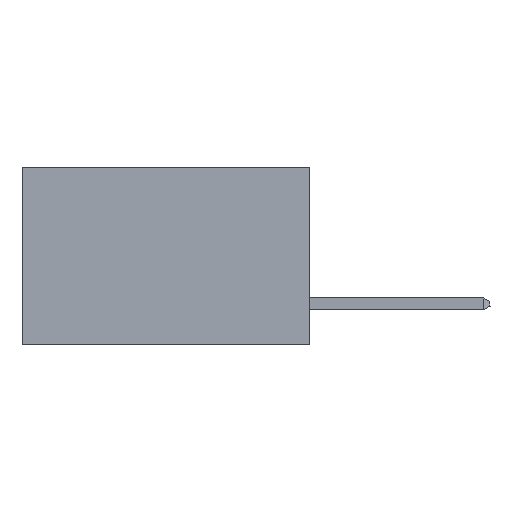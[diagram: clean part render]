
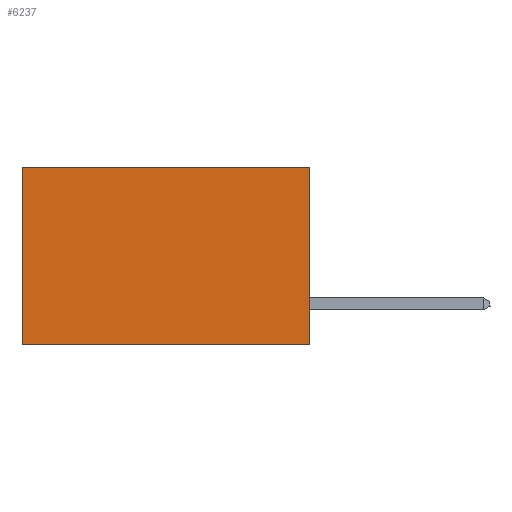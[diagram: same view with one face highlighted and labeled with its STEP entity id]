
A CAD part, left-side view. The second image highlights one B-rep face of the part: STEP entity #6237.
In plain terms, the highlighted planar face has unit normal (-1, 0, 0).
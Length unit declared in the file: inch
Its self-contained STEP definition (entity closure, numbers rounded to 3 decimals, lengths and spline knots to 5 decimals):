
#735 = EDGE_LOOP ( 'NONE', ( #9294, #25639, #48773, #8021 ) ) ;
#2298 = CARTESIAN_POINT ( 'NONE',  ( 0.2875, 0.6, -0.37 ) ) ;
#2796 = CARTESIAN_POINT ( 'NONE',  ( 0.2875, 0., 0. ) ) ;
#3446 = DIRECTION ( 'NONE',  ( 0., 0., -1. ) ) ;
#3773 = PLANE ( 'NONE',  #8908 ) ;
#4714 = LINE ( 'NONE', #18175, #43325 ) ;
#6237 = ADVANCED_FACE ( 'NONE', ( #45340 ), #3773, .F. ) ;
#6367 = CARTESIAN_POINT ( 'NONE',  ( 0.2875, 0.6, 0. ) ) ;
#7957 = CARTESIAN_POINT ( 'NONE',  ( 0.2875, 0., 0. ) ) ;
#8021 = ORIENTED_EDGE ( 'NONE', *, *, #8168, .T. ) ;
#8168 = EDGE_CURVE ( 'NONE', #41315, #24216, #46345, .T. ) ;
#8908 = AXIS2_PLACEMENT_3D ( 'NONE', #7957, #26553, #3446 ) ;
#9294 = ORIENTED_EDGE ( 'NONE', *, *, #49239, .T. ) ;
#15207 = EDGE_CURVE ( 'NONE', #41315, #23271, #4714, .T. ) ;
#16881 = CARTESIAN_POINT ( 'NONE',  ( 0.2875, 0., -0.37 ) ) ;
#17269 = EDGE_CURVE ( 'NONE', #23271, #26229, #37807, .T. ) ;
#18175 = CARTESIAN_POINT ( 'NONE',  ( 0.2875, 0., 0. ) ) ;
#21041 = VECTOR ( 'NONE', #29805, 39.37008 ) ;
#23271 = VERTEX_POINT ( 'NONE', #16881 ) ;
#24216 = VERTEX_POINT ( 'NONE', #43017 ) ;
#25639 = ORIENTED_EDGE ( 'NONE', *, *, #17269, .F. ) ;
#26229 = VERTEX_POINT ( 'NONE', #2298 ) ;
#26553 = DIRECTION ( 'NONE',  ( 1., 0., 0. ) ) ;
#29395 = LINE ( 'NONE', #6367, #34825 ) ;
#29805 = DIRECTION ( 'NONE',  ( 0., 1., 0. ) ) ;
#30519 = CARTESIAN_POINT ( 'NONE',  ( 0.2875, 0., -0.37 ) ) ;
#34825 = VECTOR ( 'NONE', #37248, 39.37008 ) ;
#37248 = DIRECTION ( 'NONE',  ( 0., 0., -1. ) ) ;
#37807 = LINE ( 'NONE', #30519, #39502 ) ;
#39502 = VECTOR ( 'NONE', #43192, 39.37008 ) ;
#41315 = VERTEX_POINT ( 'NONE', #45229 ) ;
#43017 = CARTESIAN_POINT ( 'NONE',  ( 0.2875, 0.6, 0. ) ) ;
#43192 = DIRECTION ( 'NONE',  ( 0., 1., 0. ) ) ;
#43325 = VECTOR ( 'NONE', #48746, 39.37008 ) ;
#45229 = CARTESIAN_POINT ( 'NONE',  ( 0.2875, 0., 0. ) ) ;
#45340 = FACE_OUTER_BOUND ( 'NONE', #735, .T. ) ;
#46345 = LINE ( 'NONE', #2796, #21041 ) ;
#48746 = DIRECTION ( 'NONE',  ( 0., 0., -1. ) ) ;
#48773 = ORIENTED_EDGE ( 'NONE', *, *, #15207, .F. ) ;
#49239 = EDGE_CURVE ( 'NONE', #24216, #26229, #29395, .T. ) ;
